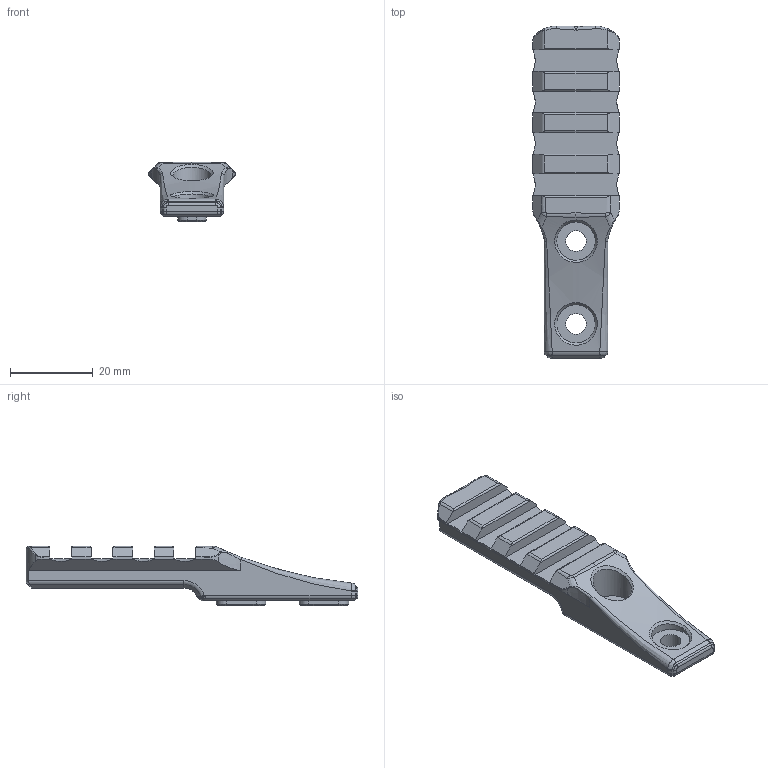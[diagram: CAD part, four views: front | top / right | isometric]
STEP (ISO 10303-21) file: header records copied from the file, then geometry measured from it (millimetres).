
FILE_DESCRIPTION(/* description */ (''),/* implementation_level */ '2;1');
FILE_NAME(/* name */ 'MLok - Picatinny Cantilever Rail.step',/* time_stamp */ '2021-06-03T20:26:42-04:00',/* author */ (''),/* organization */ (''),/* preprocessor_version */ 'ST-DEVELOPER v18.1',/* originating_system */ 'Autodesk Translation Framework v10.9.0.1377',/* authorisation */ '');
FILE_SCHEMA (('AUTOMOTIVE_DESIGN { 1 0 10303 214 3 1 1 }'));
Length unit declared in the file: millimetre
Products named in the file (1): MLok - Picatinny Cantilever Rail
Bounding box: 20.91 x 80.25 x 14.32 mm (x, y, z)
Volume: 10225.4 mm3; surface area: 4943.2 mm2
Topology: 1 solids, 1 shells, 245 faces, 599 edges, 354 vertices
Faces by surface type: bspline 87, plane 77, cylinder 57, cone 18, torus 4, sphere 2
Full cylindrical faces by diameter (mm): 5 x2, 9.3 x2
Entity records: 10000 total; most frequent: CARTESIAN_POINT 4847, ORIENTED_EDGE 1186, DIRECTION 844, EDGE_CURVE 593, VERTEX_POINT 354, AXIS2_PLACEMENT_3D 299, EDGE_LOOP 253, LINE 246
